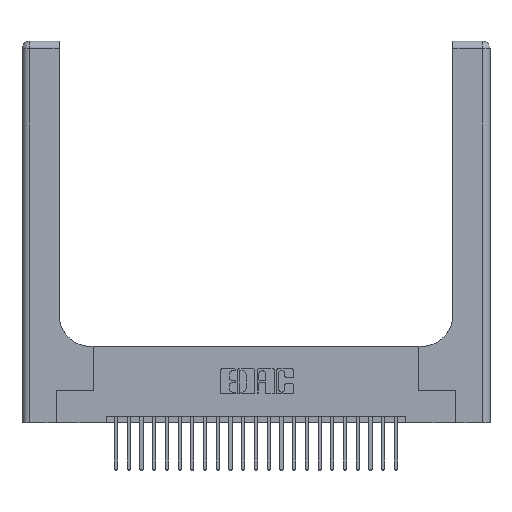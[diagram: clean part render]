
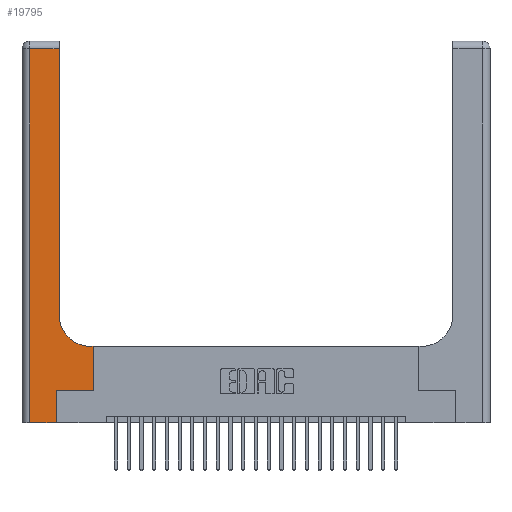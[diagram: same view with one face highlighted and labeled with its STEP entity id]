
A CAD part, top view. The second image highlights one B-rep face of the part: STEP entity #19795.
In plain terms, the highlighted planar face has unit normal (0, 0, 1).
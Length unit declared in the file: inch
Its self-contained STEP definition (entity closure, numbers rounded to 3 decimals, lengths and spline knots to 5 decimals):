
#1136 = LINE ( 'NONE', #21647, #21155 ) ;
#1188 = CARTESIAN_POINT ( 'NONE',  ( 0.06, 3., 0.37 ) ) ;
#1522 = LINE ( 'NONE', #1188, #10870 ) ;
#2020 = VERTEX_POINT ( 'NONE', #22153 ) ;
#2524 = DIRECTION ( 'NONE',  ( 0., 1., 0. ) ) ;
#3009 = ORIENTED_EDGE ( 'NONE', *, *, #11005, .T. ) ;
#3159 = ORIENTED_EDGE ( 'NONE', *, *, #11582, .T. ) ;
#3407 = VECTOR ( 'NONE', #14089, 39.37008 ) ;
#4385 = DIRECTION ( 'NONE',  ( 0., 1., 0. ) ) ;
#4388 = FACE_OUTER_BOUND ( 'NONE', #10429, .T. ) ;
#5101 = DIRECTION ( 'NONE',  ( 0., -1., 0. ) ) ;
#5107 = VECTOR ( 'NONE', #16829, 39.37008 ) ;
#5643 = CARTESIAN_POINT ( 'NONE',  ( 0.06, 0., 0.37 ) ) ;
#6326 = CARTESIAN_POINT ( 'NONE',  ( 0.2915, 3., 0.37 ) ) ;
#6550 = VECTOR ( 'NONE', #4385, 39.37008 ) ;
#6560 = DIRECTION ( 'NONE',  ( 0., 0., -1. ) ) ;
#6589 = VERTEX_POINT ( 'NONE', #15402 ) ;
#6802 = LINE ( 'NONE', #16603, #19974 ) ;
#7013 = ORIENTED_EDGE ( 'NONE', *, *, #15196, .T. ) ;
#7091 = VECTOR ( 'NONE', #12206, 39.37008 ) ;
#7501 = VERTEX_POINT ( 'NONE', #18551 ) ;
#7613 = ORIENTED_EDGE ( 'NONE', *, *, #15284, .T. ) ;
#7768 = CARTESIAN_POINT ( 'NONE',  ( 0., 3., 0.37 ) ) ;
#9042 = CIRCLE ( 'NONE', #11288, 0.25 ) ;
#9215 = VERTEX_POINT ( 'NONE', #24388 ) ;
#9412 = VERTEX_POINT ( 'NONE', #15485 ) ;
#9792 = DIRECTION ( 'NONE',  ( -1., 0., 0. ) ) ;
#10002 = VERTEX_POINT ( 'NONE', #20403 ) ;
#10018 = EDGE_CURVE ( 'NONE', #11963, #7501, #17226, .T. ) ;
#10229 = CARTESIAN_POINT ( 'NONE',  ( 0.269, 0.25, 0.37 ) ) ;
#10429 = EDGE_LOOP ( 'NONE', ( #22381, #15170, #7613, #16434, #3009, #3159, #7013, #17399, #19681 ) ) ;
#10685 = DIRECTION ( 'NONE',  ( 0., 1., 0. ) ) ;
#10772 = CARTESIAN_POINT ( 'NONE',  ( 0.269, 0., 0.37 ) ) ;
#10870 = VECTOR ( 'NONE', #5101, 39.37008 ) ;
#11005 = EDGE_CURVE ( 'NONE', #9215, #2020, #18723, .T. ) ;
#11288 = AXIS2_PLACEMENT_3D ( 'NONE', #14495, #6560, #22558 ) ;
#11582 = EDGE_CURVE ( 'NONE', #2020, #19473, #24290, .T. ) ;
#11936 = DIRECTION ( 'NONE',  ( 0., 0., -1. ) ) ;
#11963 = VERTEX_POINT ( 'NONE', #24434 ) ;
#12206 = DIRECTION ( 'NONE',  ( 1., 0., 0. ) ) ;
#12241 = CARTESIAN_POINT ( 'NONE',  ( 0., 2.94, 0.37 ) ) ;
#12355 = EDGE_CURVE ( 'NONE', #22704, #9215, #1136, .T. ) ;
#12720 = VECTOR ( 'NONE', #10685, 39.37008 ) ;
#13521 = LINE ( 'NONE', #17005, #5107 ) ;
#13611 = PLANE ( 'NONE',  #13757 ) ;
#13757 = AXIS2_PLACEMENT_3D ( 'NONE', #7768, #11936, #9792 ) ;
#14005 = EDGE_CURVE ( 'NONE', #7501, #6589, #23451, .T. ) ;
#14089 = DIRECTION ( 'NONE',  ( -1., 0., 0. ) ) ;
#14312 = CARTESIAN_POINT ( 'NONE',  ( 0.5585, 0.25, 0.37 ) ) ;
#14495 = CARTESIAN_POINT ( 'NONE',  ( 0.5415, 0.85, 0.37 ) ) ;
#15170 = ORIENTED_EDGE ( 'NONE', *, *, #14005, .T. ) ;
#15196 = EDGE_CURVE ( 'NONE', #19473, #10002, #6802, .T. ) ;
#15284 = EDGE_CURVE ( 'NONE', #6589, #22704, #1522, .T. ) ;
#15402 = CARTESIAN_POINT ( 'NONE',  ( 0.06, 2.94, 0.37 ) ) ;
#15485 = CARTESIAN_POINT ( 'NONE',  ( 0.5415, 0.6, 0.37 ) ) ;
#16434 = ORIENTED_EDGE ( 'NONE', *, *, #12355, .T. ) ;
#16603 = CARTESIAN_POINT ( 'NONE',  ( 0.5585, 0.25, 0.37 ) ) ;
#16829 = DIRECTION ( 'NONE',  ( -1., 0., 0. ) ) ;
#17005 = CARTESIAN_POINT ( 'NONE',  ( 0.2915, 0.6, 0.37 ) ) ;
#17226 = LINE ( 'NONE', #6326, #6550 ) ;
#17399 = ORIENTED_EDGE ( 'NONE', *, *, #18841, .T. ) ;
#18551 = CARTESIAN_POINT ( 'NONE',  ( 0.2915, 2.94, 0.37 ) ) ;
#18723 = LINE ( 'NONE', #10772, #12720 ) ;
#18841 = EDGE_CURVE ( 'NONE', #10002, #9412, #13521, .T. ) ;
#19473 = VERTEX_POINT ( 'NONE', #14312 ) ;
#19681 = ORIENTED_EDGE ( 'NONE', *, *, #21053, .T. ) ;
#19795 = ADVANCED_FACE ( 'NONE', ( #4388 ), #13611, .F. ) ;
#19974 = VECTOR ( 'NONE', #2524, 39.37008 ) ;
#20403 = CARTESIAN_POINT ( 'NONE',  ( 0.5585, 0.6, 0.37 ) ) ;
#21053 = EDGE_CURVE ( 'NONE', #9412, #11963, #9042, .T. ) ;
#21155 = VECTOR ( 'NONE', #23557, 39.37008 ) ;
#21647 = CARTESIAN_POINT ( 'NONE',  ( 0., 0., 0.37 ) ) ;
#22153 = CARTESIAN_POINT ( 'NONE',  ( 0.269, 0.25, 0.37 ) ) ;
#22381 = ORIENTED_EDGE ( 'NONE', *, *, #10018, .T. ) ;
#22558 = DIRECTION ( 'NONE',  ( 1., 0., 0. ) ) ;
#22704 = VERTEX_POINT ( 'NONE', #5643 ) ;
#23451 = LINE ( 'NONE', #12241, #3407 ) ;
#23557 = DIRECTION ( 'NONE',  ( 1., 0., 0. ) ) ;
#24290 = LINE ( 'NONE', #10229, #7091 ) ;
#24388 = CARTESIAN_POINT ( 'NONE',  ( 0.269, 0., 0.37 ) ) ;
#24434 = CARTESIAN_POINT ( 'NONE',  ( 0.2915, 0.85, 0.37 ) ) ;
